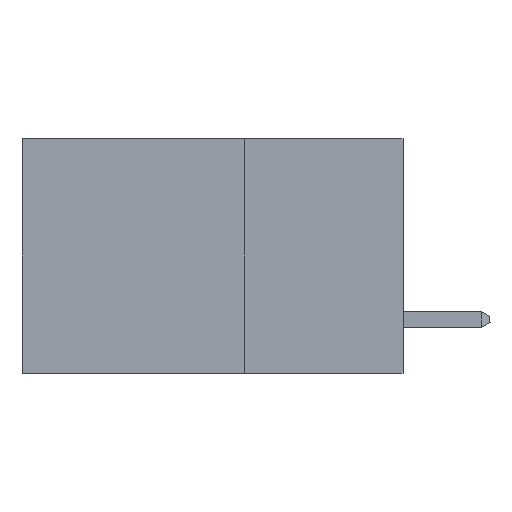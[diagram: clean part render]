
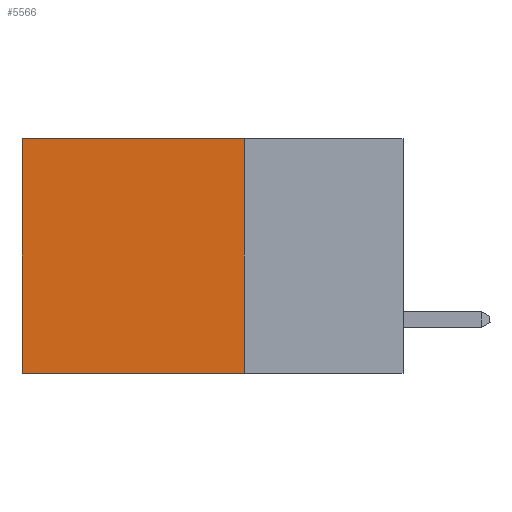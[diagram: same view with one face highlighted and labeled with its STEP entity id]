
A CAD part, left-side view. The second image highlights one B-rep face of the part: STEP entity #5566.
In plain terms, the highlighted planar face has unit normal (-1, 0, 0).
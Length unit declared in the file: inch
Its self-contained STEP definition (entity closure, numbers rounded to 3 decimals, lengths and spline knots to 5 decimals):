
#409 = ORIENTED_EDGE ( 'NONE', *, *, #1236, .T. ) ;
#750 = DIRECTION ( 'NONE',  ( 0., 1., 0. ) ) ;
#1236 = EDGE_CURVE ( 'NONE', #9874, #9056, #3142, .T. ) ;
#1416 = DIRECTION ( 'NONE',  ( 0., 0., -1. ) ) ;
#1443 = DIRECTION ( 'NONE',  ( 0., 0., -1. ) ) ;
#1503 = CARTESIAN_POINT ( 'NONE',  ( 0.2875, 0.25, -0.37 ) ) ;
#1509 = VERTEX_POINT ( 'NONE', #6994 ) ;
#1525 = CARTESIAN_POINT ( 'NONE',  ( 0.2875, 0.25, 0. ) ) ;
#1600 = DIRECTION ( 'NONE',  ( 0., 1., 0. ) ) ;
#1793 = VECTOR ( 'NONE', #1600, 39.37008 ) ;
#1947 = CARTESIAN_POINT ( 'NONE',  ( 0.2875, 0.25, 0. ) ) ;
#2184 = LINE ( 'NONE', #5418, #3991 ) ;
#2249 = VECTOR ( 'NONE', #5405, 39.37008 ) ;
#2551 = EDGE_CURVE ( 'NONE', #9874, #1509, #9356, .T. ) ;
#2713 = VECTOR ( 'NONE', #750, 39.37008 ) ;
#3079 = CARTESIAN_POINT ( 'NONE',  ( 0.2875, 0.6, -0.37 ) ) ;
#3085 = PLANE ( 'NONE',  #3707 ) ;
#3142 = LINE ( 'NONE', #6120, #1793 ) ;
#3309 = EDGE_CURVE ( 'NONE', #1509, #8419, #4630, .T. ) ;
#3707 = AXIS2_PLACEMENT_3D ( 'NONE', #1525, #7632, #1416 ) ;
#3991 = VECTOR ( 'NONE', #1443, 39.37008 ) ;
#4095 = CARTESIAN_POINT ( 'NONE',  ( 0.2875, 0.6, 0. ) ) ;
#4497 = CARTESIAN_POINT ( 'NONE',  ( 0.2875, 0.25, 0. ) ) ;
#4630 = LINE ( 'NONE', #1503, #2713 ) ;
#5405 = DIRECTION ( 'NONE',  ( 0., 0., -1. ) ) ;
#5418 = CARTESIAN_POINT ( 'NONE',  ( 0.2875, 0.6, 0. ) ) ;
#5566 = ADVANCED_FACE ( 'NONE', ( #6921 ), #3085, .F. ) ;
#6120 = CARTESIAN_POINT ( 'NONE',  ( 0.2875, 0.25, 0. ) ) ;
#6921 = FACE_OUTER_BOUND ( 'NONE', #7014, .T. ) ;
#6994 = CARTESIAN_POINT ( 'NONE',  ( 0.2875, 0.25, -0.37 ) ) ;
#7014 = EDGE_LOOP ( 'NONE', ( #9081, #9496, #9127, #409 ) ) ;
#7632 = DIRECTION ( 'NONE',  ( 1., 0., 0. ) ) ;
#8419 = VERTEX_POINT ( 'NONE', #3079 ) ;
#8430 = EDGE_CURVE ( 'NONE', #9056, #8419, #2184, .T. ) ;
#9056 = VERTEX_POINT ( 'NONE', #4095 ) ;
#9081 = ORIENTED_EDGE ( 'NONE', *, *, #8430, .T. ) ;
#9127 = ORIENTED_EDGE ( 'NONE', *, *, #2551, .F. ) ;
#9356 = LINE ( 'NONE', #4497, #2249 ) ;
#9496 = ORIENTED_EDGE ( 'NONE', *, *, #3309, .F. ) ;
#9874 = VERTEX_POINT ( 'NONE', #1947 ) ;
